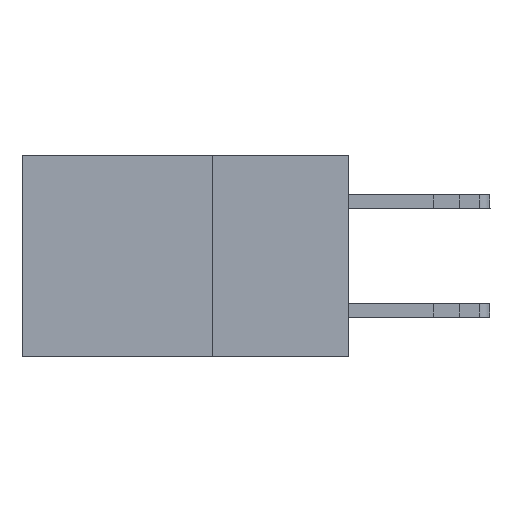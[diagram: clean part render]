
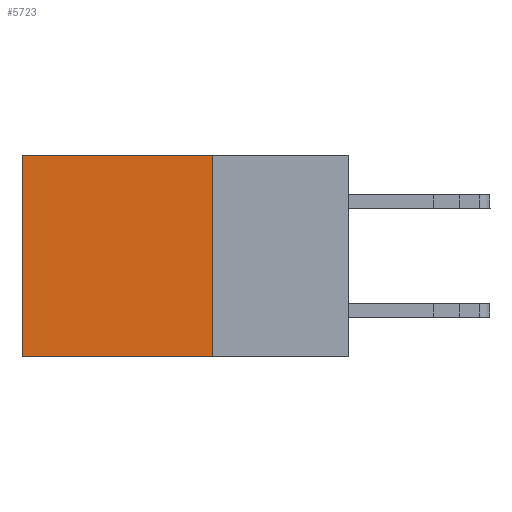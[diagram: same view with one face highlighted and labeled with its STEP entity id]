
A CAD part, left-side view. The second image highlights one B-rep face of the part: STEP entity #5723.
In plain terms, the highlighted planar face has unit normal (-1, 0, 0).
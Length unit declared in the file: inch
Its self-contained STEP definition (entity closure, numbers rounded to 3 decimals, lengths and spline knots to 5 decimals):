
#290 = EDGE_CURVE ( 'NONE', #4843, #8118, #18262, .T. ) ;
#1365 = VECTOR ( 'NONE', #16401, 39.37008 ) ;
#2042 = EDGE_CURVE ( 'NONE', #16410, #8118, #11050, .T. ) ;
#3190 = CARTESIAN_POINT ( 'NONE',  ( 0.2615, 0.6, -0.37 ) ) ;
#3317 = AXIS2_PLACEMENT_3D ( 'NONE', #9948, #18527, #18646 ) ;
#4026 = CARTESIAN_POINT ( 'NONE',  ( 0.2615, 0.6, 0. ) ) ;
#4161 = ORIENTED_EDGE ( 'NONE', *, *, #290, .F. ) ;
#4349 = PLANE ( 'NONE',  #3317 ) ;
#4843 = VERTEX_POINT ( 'NONE', #17380 ) ;
#5723 = ADVANCED_FACE ( 'NONE', ( #14949 ), #4349, .F. ) ;
#6335 = CARTESIAN_POINT ( 'NONE',  ( 0.2615, 0.25, -0.37 ) ) ;
#6348 = CARTESIAN_POINT ( 'NONE',  ( 0.2615, 0.25, 0. ) ) ;
#6542 = EDGE_LOOP ( 'NONE', ( #22777, #4161, #17865, #7842 ) ) ;
#7429 = DIRECTION ( 'NONE',  ( 0., 1., 0. ) ) ;
#7842 = ORIENTED_EDGE ( 'NONE', *, *, #20194, .T. ) ;
#8057 = VECTOR ( 'NONE', #16949, 39.37008 ) ;
#8118 = VERTEX_POINT ( 'NONE', #3190 ) ;
#8380 = LINE ( 'NONE', #6348, #20853 ) ;
#9421 = EDGE_CURVE ( 'NONE', #19721, #4843, #15386, .T. ) ;
#9948 = CARTESIAN_POINT ( 'NONE',  ( 0.2615, 0.25, -0.37 ) ) ;
#11050 = LINE ( 'NONE', #12823, #1365 ) ;
#11668 = CARTESIAN_POINT ( 'NONE',  ( 0.2615, 0.25, 0. ) ) ;
#12823 = CARTESIAN_POINT ( 'NONE',  ( 0.2615, 0.6, -0.37 ) ) ;
#14949 = FACE_OUTER_BOUND ( 'NONE', #6542, .T. ) ;
#15386 = LINE ( 'NONE', #6335, #8057 ) ;
#16401 = DIRECTION ( 'NONE',  ( 0., 0., -1. ) ) ;
#16410 = VERTEX_POINT ( 'NONE', #4026 ) ;
#16624 = VECTOR ( 'NONE', #7429, 39.37008 ) ;
#16949 = DIRECTION ( 'NONE',  ( 0., 0., -1. ) ) ;
#17380 = CARTESIAN_POINT ( 'NONE',  ( 0.2615, 0.25, -0.37 ) ) ;
#17865 = ORIENTED_EDGE ( 'NONE', *, *, #9421, .F. ) ;
#18262 = LINE ( 'NONE', #22313, #16624 ) ;
#18527 = DIRECTION ( 'NONE',  ( 1., 0., 0. ) ) ;
#18646 = DIRECTION ( 'NONE',  ( 0., 0., -1. ) ) ;
#19721 = VERTEX_POINT ( 'NONE', #11668 ) ;
#20194 = EDGE_CURVE ( 'NONE', #19721, #16410, #8380, .T. ) ;
#20853 = VECTOR ( 'NONE', #21224, 39.37008 ) ;
#21224 = DIRECTION ( 'NONE',  ( 0., 1., 0. ) ) ;
#22313 = CARTESIAN_POINT ( 'NONE',  ( 0.2615, 0.25, -0.37 ) ) ;
#22777 = ORIENTED_EDGE ( 'NONE', *, *, #2042, .T. ) ;
